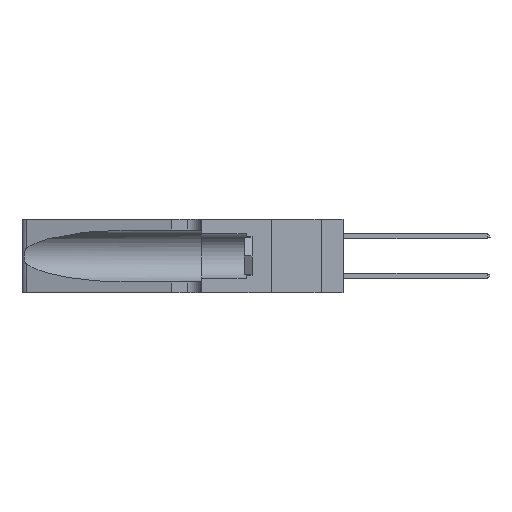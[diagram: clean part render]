
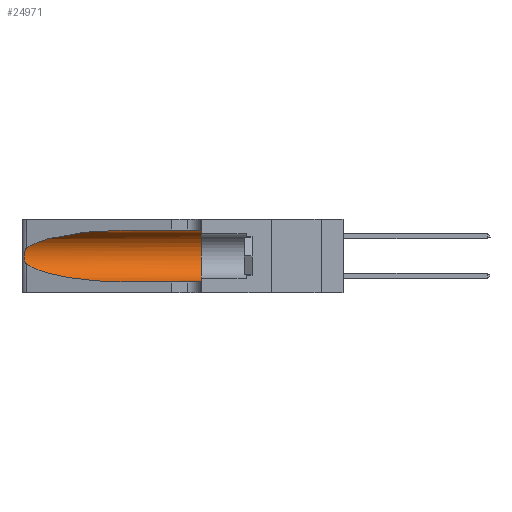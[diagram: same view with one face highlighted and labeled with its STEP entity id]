
A CAD part, left-side view. The second image highlights one B-rep face of the part: STEP entity #24971.
In plain terms, the highlighted cylindrical face has radius 3.308 mm (diameter 6.617 mm), a partial arc.
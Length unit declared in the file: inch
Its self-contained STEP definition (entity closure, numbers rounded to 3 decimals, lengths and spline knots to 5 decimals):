
#2011 = VERTEX_POINT ( 'NONE', #5989 ) ;
#2462 = CARTESIAN_POINT ( 'NONE',  ( 0.1305, 0.35, 0.185 ) ) ;
#3278 = CARTESIAN_POINT ( 'NONE',  ( 0.25487, 1.22718, 0.22369 ) ) ;
#5549 = LINE ( 'NONE', #15105, #13207 ) ;
#5620 = CARTESIAN_POINT ( 'NONE',  ( 0.25555, 1.22994, 0.2215 ) ) ;
#5989 = CARTESIAN_POINT ( 'NONE',  ( 0.1305, 0.72297, 0.31525 ) ) ;
#6238 = DIRECTION ( 'NONE',  ( 0., 0., 1. ) ) ;
#6446 = EDGE_CURVE ( 'NONE', #36746, #22212, #5549, .T. ) ;
#6538 = ORIENTED_EDGE ( 'NONE', *, *, #8295, .F. ) ;
#7243 = CARTESIAN_POINT ( 'NONE',  ( 0.1305, 0.72297, 0.31525 ) ) ;
#7413 = DIRECTION ( 'NONE',  ( 0., 0., -1. ) ) ;
#8295 = EDGE_CURVE ( 'NONE', #8983, #22212, #17070, .T. ) ;
#8983 = VERTEX_POINT ( 'NONE', #25878 ) ;
#9393 = EDGE_CURVE ( 'NONE', #31199, #39144, #10397, .T. ) ;
#9409 = CARTESIAN_POINT ( 'NONE',  ( 0.25639, 1.23186, 0.15144 ) ) ;
#10397 = B_SPLINE_CURVE_WITH_KNOTS ( 'NONE', 3,
 ( #28141, #5620, #20584, #35839, #35343, #24524, #39286, #16321, #46906, #42944, #31880, #9409, #35665, #20750 ),
 .UNSPECIFIED., .F., .F.,
 ( 4, 2, 2, 2, 2, 2, 4 ),
 ( 0., 0.00027, 0.00053, 0.00107, 0.0016, 0.00187, 0.00214 ),
 .UNSPECIFIED. ) ;
#12650 = ORIENTED_EDGE ( 'NONE', *, *, #9393, .T. ) ;
#13207 = VECTOR ( 'NONE', #37761, 39.37008 ) ;
#15037 = ORIENTED_EDGE ( 'NONE', *, *, #46466, .T. ) ;
#15091 = CARTESIAN_POINT ( 'NONE',  ( 0.1305, 1.61858, 0.31525 ) ) ;
#15105 = CARTESIAN_POINT ( 'NONE',  ( 0.1305, 1.61858, 0.05475 ) ) ;
#16120 = CARTESIAN_POINT ( 'NONE',  ( 0.25487, 1.22718, 0.14631 ) ) ;
#16321 = CARTESIAN_POINT ( 'NONE',  ( 0.26075, 1.23896, 0.178 ) ) ;
#17070 = CIRCLE ( 'NONE', #32834, 0.13025 ) ;
#18939 = CARTESIAN_POINT ( 'NONE',  ( 0.1305, 0.72297, 0.05475 ) ) ;
#19309 = EDGE_CURVE ( 'NONE', #2011, #31199, #20376, .T. ) ;
#20376 =( BOUNDED_CURVE ( )  B_SPLINE_CURVE ( 3, ( #7243, #21877, #37130, #41246 ),
 .UNSPECIFIED., .F., .T. ) 
 B_SPLINE_CURVE_WITH_KNOTS ( ( 4, 4 ),
 ( 1.5708, 2.84003 ),
 .UNSPECIFIED. ) 
 CURVE ( )  GEOMETRIC_REPRESENTATION_ITEM ( )  RATIONAL_B_SPLINE_CURVE ( ( 1., 0.87, 0.87, 1. ) ) 
 REPRESENTATION_ITEM ( '' )  );
#20584 = CARTESIAN_POINT ( 'NONE',  ( 0.25639, 1.23184, 0.21858 ) ) ;
#20750 = CARTESIAN_POINT ( 'NONE',  ( 0.25487, 1.22718, 0.14631 ) ) ;
#21706 = EDGE_LOOP ( 'NONE', ( #43964, #12650, #15037, #41879, #6538, #48599 ) ) ;
#21877 = CARTESIAN_POINT ( 'NONE',  ( 0.18966, 0.96281, 0.31525 ) ) ;
#22212 = VERTEX_POINT ( 'NONE', #32112 ) ;
#22499 = DIRECTION ( 'NONE',  ( 0., -1., 0. ) ) ;
#23358 = CARTESIAN_POINT ( 'NONE',  ( 0.2373, 1.15595, 0.08982 ) ) ;
#24524 = CARTESIAN_POINT ( 'NONE',  ( 0.26018, 1.23835, 0.19895 ) ) ;
#24971 = ADVANCED_FACE ( 'NONE', ( #25022 ), #34412, .F. ) ;
#25022 = FACE_OUTER_BOUND ( 'NONE', #21706, .T. ) ;
#25878 = CARTESIAN_POINT ( 'NONE',  ( 0.1305, 0.35, 0.31525 ) ) ;
#26770 = LINE ( 'NONE', #15091, #39085 ) ;
#27454 = CARTESIAN_POINT ( 'NONE',  ( 0.18966, 0.96281, 0.05475 ) ) ;
#28075 = EDGE_CURVE ( 'NONE', #2011, #8983, #26770, .T. ) ;
#28141 = CARTESIAN_POINT ( 'NONE',  ( 0.25487, 1.22718, 0.22369 ) ) ;
#28750 = DIRECTION ( 'NONE',  ( 0., 1., 0. ) ) ;
#31199 = VERTEX_POINT ( 'NONE', #3278 ) ;
#31880 = CARTESIAN_POINT ( 'NONE',  ( 0.25789, 1.23486, 0.15765 ) ) ;
#32112 = CARTESIAN_POINT ( 'NONE',  ( 0.1305, 0.35, 0.05475 ) ) ;
#32814 = AXIS2_PLACEMENT_3D ( 'NONE', #48370, #41074, #7413 ) ;
#32834 = AXIS2_PLACEMENT_3D ( 'NONE', #2462, #28750, #6238 ) ;
#34412 = CYLINDRICAL_SURFACE ( 'NONE', #32814, 0.13025 ) ;
#35343 = CARTESIAN_POINT ( 'NONE',  ( 0.25854, 1.2359, 0.20912 ) ) ;
#35665 = CARTESIAN_POINT ( 'NONE',  ( 0.25555, 1.22993, 0.14849 ) ) ;
#35839 = CARTESIAN_POINT ( 'NONE',  ( 0.25787, 1.23484, 0.2124 ) ) ;
#36746 = VERTEX_POINT ( 'NONE', #18939 ) ;
#37130 = CARTESIAN_POINT ( 'NONE',  ( 0.2373, 1.15595, 0.28018 ) ) ;
#37761 = DIRECTION ( 'NONE',  ( 0., -1., 0. ) ) ;
#39085 = VECTOR ( 'NONE', #22499, 39.37008 ) ;
#39144 = VERTEX_POINT ( 'NONE', #41213 ) ;
#39286 = CARTESIAN_POINT ( 'NONE',  ( 0.26075, 1.23896, 0.19203 ) ) ;
#39433 = CARTESIAN_POINT ( 'NONE',  ( 0.1305, 0.72297, 0.05475 ) ) ;
#40818 =( BOUNDED_CURVE ( )  B_SPLINE_CURVE ( 3, ( #16120, #23358, #27454, #39433 ),
 .UNSPECIFIED., .F., .T. ) 
 B_SPLINE_CURVE_WITH_KNOTS ( ( 4, 4 ),
 ( 3.44316, 4.71239 ),
 .UNSPECIFIED. ) 
 CURVE ( )  GEOMETRIC_REPRESENTATION_ITEM ( )  RATIONAL_B_SPLINE_CURVE ( ( 1., 0.87, 0.87, 1. ) ) 
 REPRESENTATION_ITEM ( '' )  );
#41074 = DIRECTION ( 'NONE',  ( 0., -1., 0. ) ) ;
#41213 = CARTESIAN_POINT ( 'NONE',  ( 0.25487, 1.22718, 0.14631 ) ) ;
#41246 = CARTESIAN_POINT ( 'NONE',  ( 0.25487, 1.22718, 0.22369 ) ) ;
#41879 = ORIENTED_EDGE ( 'NONE', *, *, #6446, .T. ) ;
#42944 = CARTESIAN_POINT ( 'NONE',  ( 0.25856, 1.23593, 0.16098 ) ) ;
#43964 = ORIENTED_EDGE ( 'NONE', *, *, #19309, .T. ) ;
#46466 = EDGE_CURVE ( 'NONE', #39144, #36746, #40818, .T. ) ;
#46906 = CARTESIAN_POINT ( 'NONE',  ( 0.26017, 1.23833, 0.17102 ) ) ;
#48370 = CARTESIAN_POINT ( 'NONE',  ( 0.1305, 1.61858, 0.185 ) ) ;
#48599 = ORIENTED_EDGE ( 'NONE', *, *, #28075, .F. ) ;
